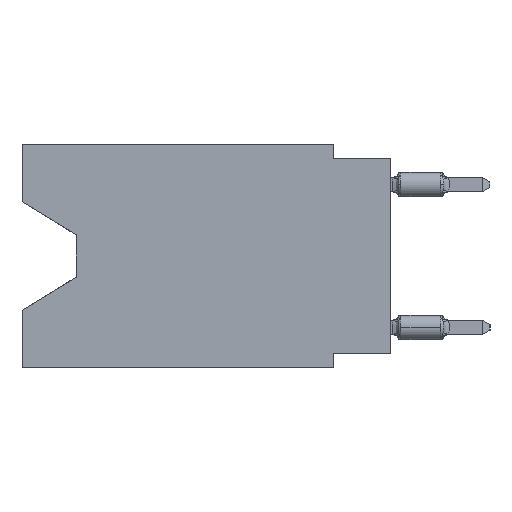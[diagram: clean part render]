
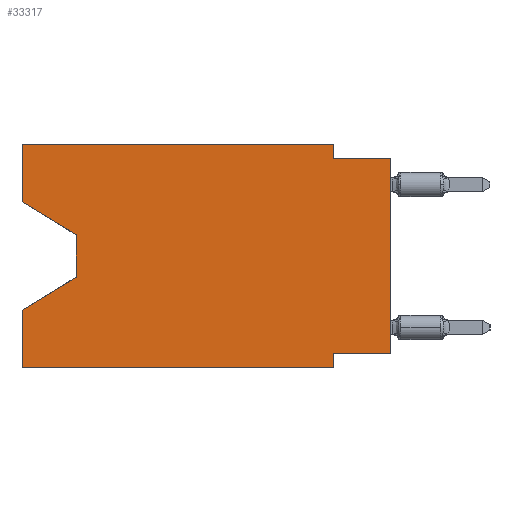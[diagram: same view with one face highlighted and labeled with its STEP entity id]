
A CAD part, left-side view. The second image highlights one B-rep face of the part: STEP entity #33317.
In plain terms, the highlighted planar face has unit normal (-1, 0, 0).
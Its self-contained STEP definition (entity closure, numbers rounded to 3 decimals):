
#84 = VERTEX_POINT ( 'NONE', #16512 ) ;
#588 = CARTESIAN_POINT ( 'NONE',  ( 0., 13.97, -4.013 ) ) ;
#1033 = CARTESIAN_POINT ( 'NONE',  ( 0., 2.54, -9.906 ) ) ;
#1932 = EDGE_CURVE ( 'NONE', #3430, #3571, #35389, .T. ) ;
#2008 = VECTOR ( 'NONE', #36036, 1000. ) ;
#2222 = ORIENTED_EDGE ( 'NONE', *, *, #25292, .F. ) ;
#2767 = CARTESIAN_POINT ( 'NONE',  ( 0., 16.383, 0. ) ) ;
#2811 = VECTOR ( 'NONE', #9337, 1000. ) ;
#3048 = EDGE_CURVE ( 'NONE', #5996, #22187, #5650, .T. ) ;
#3199 = VERTEX_POINT ( 'NONE', #35766 ) ;
#3430 = VERTEX_POINT ( 'NONE', #8581 ) ;
#3571 = VERTEX_POINT ( 'NONE', #34798 ) ;
#4008 = ORIENTED_EDGE ( 'NONE', *, *, #17611, .F. ) ;
#4151 = CARTESIAN_POINT ( 'NONE',  ( 0., 16.383, 0. ) ) ;
#5338 = DIRECTION ( 'NONE',  ( 1., 0., 0. ) ) ;
#5341 = CARTESIAN_POINT ( 'NONE',  ( 0., 13.97, -4.013 ) ) ;
#5449 = EDGE_CURVE ( 'NONE', #25856, #17152, #20845, .T. ) ;
#5650 = LINE ( 'NONE', #8446, #2008 ) ;
#5996 = VERTEX_POINT ( 'NONE', #8938 ) ;
#6073 = EDGE_LOOP ( 'NONE', ( #23873, #21816, #26702, #12295, #25568, #31679, #4008, #31309, #10494, #8002, #6453, #2222 ) ) ;
#6328 = EDGE_CURVE ( 'NONE', #3199, #84, #25086, .T. ) ;
#6453 = ORIENTED_EDGE ( 'NONE', *, *, #27631, .F. ) ;
#6531 = DIRECTION ( 'NONE',  ( 0., -0.855, -0.519 ) ) ;
#7295 = CARTESIAN_POINT ( 'NONE',  ( 0., 13.97, -5.893 ) ) ;
#7512 = VECTOR ( 'NONE', #34801, 1000. ) ;
#8002 = ORIENTED_EDGE ( 'NONE', *, *, #24212, .F. ) ;
#8162 = DIRECTION ( 'NONE',  ( 0., 0., 1. ) ) ;
#8446 = CARTESIAN_POINT ( 'NONE',  ( 0., 2.54, -9.906 ) ) ;
#8513 = VECTOR ( 'NONE', #27011, 1000. ) ;
#8581 = CARTESIAN_POINT ( 'NONE',  ( 0., 13.97, -5.893 ) ) ;
#8938 = CARTESIAN_POINT ( 'NONE',  ( 0., 2.54, -9.271 ) ) ;
#9337 = DIRECTION ( 'NONE',  ( 0., 0., -1. ) ) ;
#9415 = VECTOR ( 'NONE', #15506, 1000. ) ;
#9491 = CARTESIAN_POINT ( 'NONE',  ( 0., 16.383, -2.546 ) ) ;
#9512 = LINE ( 'NONE', #9874, #31279 ) ;
#9874 = CARTESIAN_POINT ( 'NONE',  ( 0., 0., -9.271 ) ) ;
#9938 = VECTOR ( 'NONE', #11098, 1000. ) ;
#10377 = DIRECTION ( 'NONE',  ( 0., 0., -1. ) ) ;
#10494 = ORIENTED_EDGE ( 'NONE', *, *, #31524, .F. ) ;
#10590 = LINE ( 'NONE', #2767, #14636 ) ;
#11098 = DIRECTION ( 'NONE',  ( 0., -1., 0. ) ) ;
#11748 = VERTEX_POINT ( 'NONE', #24481 ) ;
#12098 = LINE ( 'NONE', #23460, #7512 ) ;
#12295 = ORIENTED_EDGE ( 'NONE', *, *, #32219, .F. ) ;
#13042 = VECTOR ( 'NONE', #33857, 1000. ) ;
#13093 = CARTESIAN_POINT ( 'NONE',  ( 0., 16.383, -2.546 ) ) ;
#13325 = VERTEX_POINT ( 'NONE', #23720 ) ;
#13709 = FACE_OUTER_BOUND ( 'NONE', #6073, .T. ) ;
#13912 = CARTESIAN_POINT ( 'NONE',  ( 0., 0., 0. ) ) ;
#13979 = VECTOR ( 'NONE', #10377, 1000. ) ;
#14636 = VECTOR ( 'NONE', #22677, 1000. ) ;
#15506 = DIRECTION ( 'NONE',  ( 0., 0., 1. ) ) ;
#16512 = CARTESIAN_POINT ( 'NONE',  ( 0., 0., -0.635 ) ) ;
#16785 = VERTEX_POINT ( 'NONE', #33850 ) ;
#16940 = AXIS2_PLACEMENT_3D ( 'NONE', #33616, #5338, #31189 ) ;
#17152 = VERTEX_POINT ( 'NONE', #5341 ) ;
#17611 = EDGE_CURVE ( 'NONE', #3199, #5996, #9512, .T. ) ;
#18283 = LINE ( 'NONE', #4151, #9415 ) ;
#18428 = DIRECTION ( 'NONE',  ( 0., 1., 0. ) ) ;
#18987 = LINE ( 'NONE', #21963, #13042 ) ;
#20845 = LINE ( 'NONE', #9491, #24005 ) ;
#21816 = ORIENTED_EDGE ( 'NONE', *, *, #29044, .T. ) ;
#21963 = CARTESIAN_POINT ( 'NONE',  ( 0., 16.383, -9.906 ) ) ;
#22187 = VERTEX_POINT ( 'NONE', #1033 ) ;
#22677 = DIRECTION ( 'NONE',  ( 0., -1., 0. ) ) ;
#23208 = CARTESIAN_POINT ( 'NONE',  ( 0., 2.54, -0.635 ) ) ;
#23460 = CARTESIAN_POINT ( 'NONE',  ( 0., 16.383, 0. ) ) ;
#23666 = LINE ( 'NONE', #588, #2811 ) ;
#23720 = CARTESIAN_POINT ( 'NONE',  ( 0., 16.383, 0. ) ) ;
#23873 = ORIENTED_EDGE ( 'NONE', *, *, #5449, .T. ) ;
#24005 = VECTOR ( 'NONE', #6531, 1000. ) ;
#24212 = EDGE_CURVE ( 'NONE', #16785, #31733, #29354, .T. ) ;
#24481 = CARTESIAN_POINT ( 'NONE',  ( 0., 16.383, -9.906 ) ) ;
#25086 = LINE ( 'NONE', #13912, #30948 ) ;
#25292 = EDGE_CURVE ( 'NONE', #25856, #13325, #12098, .T. ) ;
#25568 = ORIENTED_EDGE ( 'NONE', *, *, #34549, .T. ) ;
#25856 = VERTEX_POINT ( 'NONE', #13093 ) ;
#26586 = CARTESIAN_POINT ( 'NONE',  ( 0., 2.54, 0. ) ) ;
#26702 = ORIENTED_EDGE ( 'NONE', *, *, #1932, .T. ) ;
#27011 = DIRECTION ( 'NONE',  ( 0., 0.855, -0.519 ) ) ;
#27631 = EDGE_CURVE ( 'NONE', #13325, #16785, #10590, .T. ) ;
#29044 = EDGE_CURVE ( 'NONE', #17152, #3430, #23666, .T. ) ;
#29354 = LINE ( 'NONE', #26586, #13979 ) ;
#30625 = LINE ( 'NONE', #33799, #9938 ) ;
#30948 = VECTOR ( 'NONE', #8162, 1000. ) ;
#31189 = DIRECTION ( 'NONE',  ( 0., 0., -1. ) ) ;
#31279 = VECTOR ( 'NONE', #18428, 1000. ) ;
#31309 = ORIENTED_EDGE ( 'NONE', *, *, #6328, .T. ) ;
#31524 = EDGE_CURVE ( 'NONE', #31733, #84, #30625, .T. ) ;
#31679 = ORIENTED_EDGE ( 'NONE', *, *, #3048, .F. ) ;
#31733 = VERTEX_POINT ( 'NONE', #23208 ) ;
#32219 = EDGE_CURVE ( 'NONE', #11748, #3571, #18283, .T. ) ;
#33317 = ADVANCED_FACE ( 'NONE', ( #13709 ), #34359, .F. ) ;
#33616 = CARTESIAN_POINT ( 'NONE',  ( 0., 16.383, 0. ) ) ;
#33799 = CARTESIAN_POINT ( 'NONE',  ( 0., 0., -0.635 ) ) ;
#33850 = CARTESIAN_POINT ( 'NONE',  ( 0., 2.54, 0. ) ) ;
#33857 = DIRECTION ( 'NONE',  ( 0., -1., 0. ) ) ;
#34359 = PLANE ( 'NONE',  #16940 ) ;
#34549 = EDGE_CURVE ( 'NONE', #11748, #22187, #18987, .T. ) ;
#34798 = CARTESIAN_POINT ( 'NONE',  ( 0., 16.383, -7.36 ) ) ;
#34801 = DIRECTION ( 'NONE',  ( 0., 0., 1. ) ) ;
#35389 = LINE ( 'NONE', #7295, #8513 ) ;
#35766 = CARTESIAN_POINT ( 'NONE',  ( 0., 0., -9.271 ) ) ;
#36036 = DIRECTION ( 'NONE',  ( 0., 0., -1. ) ) ;
